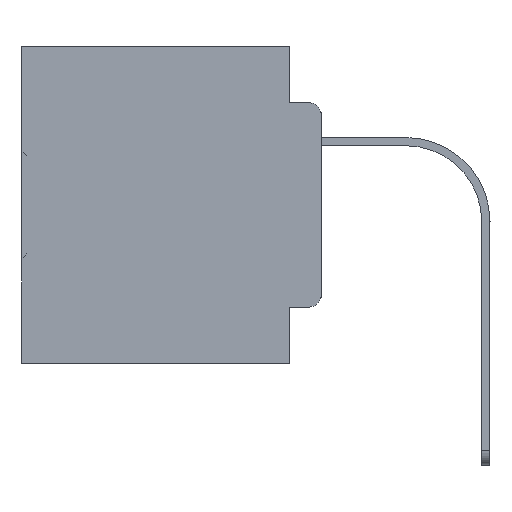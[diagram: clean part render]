
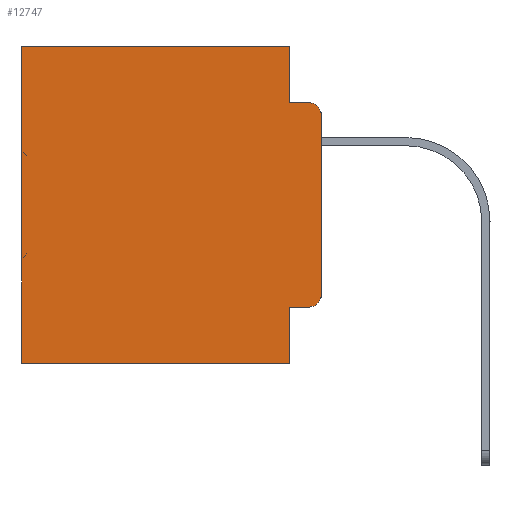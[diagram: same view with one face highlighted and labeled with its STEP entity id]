
A CAD part, left-side view. The second image highlights one B-rep face of the part: STEP entity #12747.
In plain terms, the highlighted planar face has unit normal (-1, 0, 0).
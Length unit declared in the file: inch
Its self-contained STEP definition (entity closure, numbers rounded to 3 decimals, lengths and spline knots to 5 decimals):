
#142 = ORIENTED_EDGE ( 'NONE', *, *, #22097, .T. ) ;
#545 = CARTESIAN_POINT ( 'NONE',  ( 0.298, 0., -0.5 ) ) ;
#614 = VECTOR ( 'NONE', #8872, 39.37008 ) ;
#838 = PLANE ( 'NONE',  #26111 ) ;
#1212 = LINE ( 'NONE', #17877, #11146 ) ;
#1815 = LINE ( 'NONE', #6614, #31631 ) ;
#3027 = LINE ( 'NONE', #545, #614 ) ;
#3399 = VERTEX_POINT ( 'NONE', #11410 ) ;
#3920 = LINE ( 'NONE', #6910, #29075 ) ;
#4652 = VECTOR ( 'NONE', #21542, 39.37008 ) ;
#4713 = LINE ( 'NONE', #28704, #9102 ) ;
#4783 = DIRECTION ( 'NONE',  ( 0., 0., -1. ) ) ;
#5928 = CARTESIAN_POINT ( 'NONE',  ( 0.298, 0.051, -0.5 ) ) ;
#6372 = CARTESIAN_POINT ( 'NONE',  ( 0.298, 0.473, 0. ) ) ;
#6614 = CARTESIAN_POINT ( 'NONE',  ( 0.298, 0., 0. ) ) ;
#6910 = CARTESIAN_POINT ( 'NONE',  ( 0.298, 0.051, -0.0885 ) ) ;
#6972 = CARTESIAN_POINT ( 'NONE',  ( 0.298, 0.473, 0. ) ) ;
#7125 = VERTEX_POINT ( 'NONE', #16606 ) ;
#7436 = DIRECTION ( 'NONE',  ( -1., 0., 0. ) ) ;
#7576 = CARTESIAN_POINT ( 'NONE',  ( 0.298, 0.051, -0.0885 ) ) ;
#8623 = LINE ( 'NONE', #32781, #23650 ) ;
#8630 = CARTESIAN_POINT ( 'NONE',  ( 0.298, 0., 0. ) ) ;
#8872 = DIRECTION ( 'NONE',  ( 0., 1., 0. ) ) ;
#9102 = VECTOR ( 'NONE', #22836, 39.37008 ) ;
#10134 = VECTOR ( 'NONE', #34144, 39.37008 ) ;
#10711 = CARTESIAN_POINT ( 'NONE',  ( 0.298, 0., 0. ) ) ;
#11146 = VECTOR ( 'NONE', #22853, 39.37008 ) ;
#11376 = VERTEX_POINT ( 'NONE', #5928 ) ;
#11410 = CARTESIAN_POINT ( 'NONE',  ( 0.298, 0.051, 0. ) ) ;
#11424 = CARTESIAN_POINT ( 'NONE',  ( 0.298, 0., -0.1085 ) ) ;
#12082 = DIRECTION ( 'NONE',  ( 0., -1., 0. ) ) ;
#12747 = ADVANCED_FACE ( 'NONE', ( #27472 ), #838, .F. ) ;
#12932 = CIRCLE ( 'NONE', #28267, 0.02 ) ;
#13444 = EDGE_LOOP ( 'NONE', ( #18273, #142, #14808, #16770, #34828, #28582, #34581, #29916, #28836, #34238 ) ) ;
#13614 = DIRECTION ( 'NONE',  ( 0., -1., 0. ) ) ;
#13738 = LINE ( 'NONE', #10711, #4652 ) ;
#14808 = ORIENTED_EDGE ( 'NONE', *, *, #14997, .F. ) ;
#14997 = EDGE_CURVE ( 'NONE', #19964, #30525, #3920, .T. ) ;
#16072 = VERTEX_POINT ( 'NONE', #29388 ) ;
#16606 = CARTESIAN_POINT ( 'NONE',  ( 0.298, 0.051, -0.4115 ) ) ;
#16770 = ORIENTED_EDGE ( 'NONE', *, *, #18535, .F. ) ;
#16995 = DIRECTION ( 'NONE',  ( 1., 0., 0. ) ) ;
#17877 = CARTESIAN_POINT ( 'NONE',  ( 0.298, 0.051, 0. ) ) ;
#18243 = CIRCLE ( 'NONE', #22776, 0.02 ) ;
#18273 = ORIENTED_EDGE ( 'NONE', *, *, #22287, .F. ) ;
#18535 = EDGE_CURVE ( 'NONE', #3399, #19964, #4713, .T. ) ;
#19964 = VERTEX_POINT ( 'NONE', #7576 ) ;
#20445 = VERTEX_POINT ( 'NONE', #27232 ) ;
#20593 = VERTEX_POINT ( 'NONE', #11424 ) ;
#20916 = EDGE_CURVE ( 'NONE', #11376, #16072, #3027, .T. ) ;
#21542 = DIRECTION ( 'NONE',  ( 0., 0., -1. ) ) ;
#22097 = EDGE_CURVE ( 'NONE', #20593, #30525, #18243, .T. ) ;
#22287 = EDGE_CURVE ( 'NONE', #20593, #24447, #13738, .T. ) ;
#22483 = CARTESIAN_POINT ( 'NONE',  ( 0.298, 0.02, -0.0885 ) ) ;
#22776 = AXIS2_PLACEMENT_3D ( 'NONE', #26518, #31844, #26693 ) ;
#22836 = DIRECTION ( 'NONE',  ( 0., 0., -1. ) ) ;
#22853 = DIRECTION ( 'NONE',  ( 0., 0., -1. ) ) ;
#23136 = DIRECTION ( 'NONE',  ( 0., 0., -1. ) ) ;
#23650 = VECTOR ( 'NONE', #13614, 39.37008 ) ;
#24447 = VERTEX_POINT ( 'NONE', #27770 ) ;
#25446 = EDGE_CURVE ( 'NONE', #7125, #11376, #1212, .T. ) ;
#26111 = AXIS2_PLACEMENT_3D ( 'NONE', #8630, #16995, #23136 ) ;
#26164 = LINE ( 'NONE', #6972, #10134 ) ;
#26518 = CARTESIAN_POINT ( 'NONE',  ( 0.298, 0.02, -0.1085 ) ) ;
#26693 = DIRECTION ( 'NONE',  ( 0., 0., -1. ) ) ;
#27232 = CARTESIAN_POINT ( 'NONE',  ( 0.298, 0.02, -0.4115 ) ) ;
#27472 = FACE_OUTER_BOUND ( 'NONE', #13444, .T. ) ;
#27770 = CARTESIAN_POINT ( 'NONE',  ( 0.298, 0., -0.3915 ) ) ;
#28267 = AXIS2_PLACEMENT_3D ( 'NONE', #31778, #7436, #4783 ) ;
#28582 = ORIENTED_EDGE ( 'NONE', *, *, #34434, .T. ) ;
#28704 = CARTESIAN_POINT ( 'NONE',  ( 0.298, 0.051, 0. ) ) ;
#28821 = DIRECTION ( 'NONE',  ( 0., 1., 0. ) ) ;
#28836 = ORIENTED_EDGE ( 'NONE', *, *, #32364, .T. ) ;
#29075 = VECTOR ( 'NONE', #12082, 39.37008 ) ;
#29388 = CARTESIAN_POINT ( 'NONE',  ( 0.298, 0.473, -0.5 ) ) ;
#29916 = ORIENTED_EDGE ( 'NONE', *, *, #25446, .F. ) ;
#30114 = VERTEX_POINT ( 'NONE', #6372 ) ;
#30525 = VERTEX_POINT ( 'NONE', #22483 ) ;
#31340 = EDGE_CURVE ( 'NONE', #3399, #30114, #1815, .T. ) ;
#31631 = VECTOR ( 'NONE', #28821, 39.37008 ) ;
#31778 = CARTESIAN_POINT ( 'NONE',  ( 0.298, 0.02, -0.3915 ) ) ;
#31844 = DIRECTION ( 'NONE',  ( -1., 0., 0. ) ) ;
#32364 = EDGE_CURVE ( 'NONE', #7125, #20445, #8623, .T. ) ;
#32781 = CARTESIAN_POINT ( 'NONE',  ( 0.298, 0.051, -0.4115 ) ) ;
#33224 = EDGE_CURVE ( 'NONE', #20445, #24447, #12932, .T. ) ;
#34144 = DIRECTION ( 'NONE',  ( 0., 0., -1. ) ) ;
#34238 = ORIENTED_EDGE ( 'NONE', *, *, #33224, .T. ) ;
#34434 = EDGE_CURVE ( 'NONE', #30114, #16072, #26164, .T. ) ;
#34581 = ORIENTED_EDGE ( 'NONE', *, *, #20916, .F. ) ;
#34828 = ORIENTED_EDGE ( 'NONE', *, *, #31340, .T. ) ;
